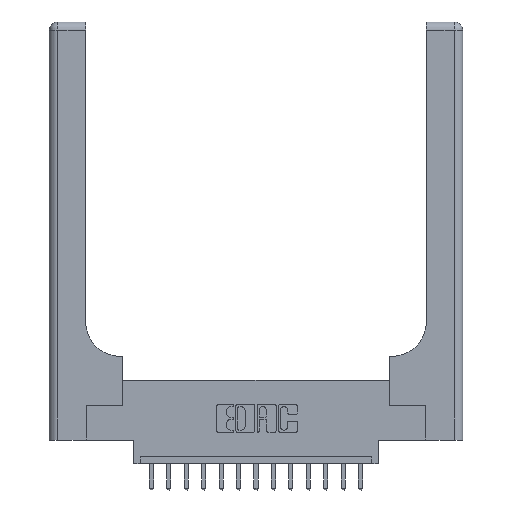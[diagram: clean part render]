
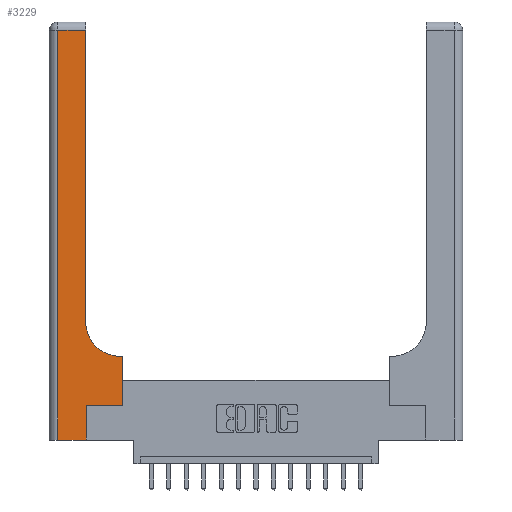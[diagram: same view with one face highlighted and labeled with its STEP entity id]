
A CAD part, top view. The second image highlights one B-rep face of the part: STEP entity #3229.
In plain terms, the highlighted planar face has unit normal (0, 0, 1).
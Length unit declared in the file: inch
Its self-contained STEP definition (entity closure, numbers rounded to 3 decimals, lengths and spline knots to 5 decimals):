
#94 = EDGE_CURVE ( 'NONE', #2724, #3836, #13927, .T. ) ;
#592 = ORIENTED_EDGE ( 'NONE', *, *, #8677, .T. ) ;
#662 = EDGE_CURVE ( 'NONE', #2136, #1271, #756, .T. ) ;
#756 = LINE ( 'NONE', #15656, #7373 ) ;
#809 = CARTESIAN_POINT ( 'NONE',  ( 0.265, 0.25, 0.37 ) ) ;
#1271 = VERTEX_POINT ( 'NONE', #15515 ) ;
#1373 = DIRECTION ( 'NONE',  ( 0., 1., 0. ) ) ;
#1915 = VERTEX_POINT ( 'NONE', #5885 ) ;
#1947 = VECTOR ( 'NONE', #14569, 39.37008 ) ;
#2000 = ORIENTED_EDGE ( 'NONE', *, *, #14840, .T. ) ;
#2136 = VERTEX_POINT ( 'NONE', #6318 ) ;
#2673 = ORIENTED_EDGE ( 'NONE', *, *, #662, .T. ) ;
#2724 = VERTEX_POINT ( 'NONE', #8294 ) ;
#2776 = EDGE_LOOP ( 'NONE', ( #4238, #15175, #2673, #2000, #15397, #592, #6553, #10457, #15063 ) ) ;
#3229 = ADVANCED_FACE ( 'NONE', ( #16634 ), #5889, .F. ) ;
#3540 = CARTESIAN_POINT ( 'NONE',  ( 0.528, 0.25, 0.37 ) ) ;
#3836 = VERTEX_POINT ( 'NONE', #5038 ) ;
#3899 = EDGE_CURVE ( 'NONE', #4764, #2724, #15065, .T. ) ;
#4098 = LINE ( 'NONE', #9790, #9730 ) ;
#4238 = ORIENTED_EDGE ( 'NONE', *, *, #11075, .T. ) ;
#4522 = DIRECTION ( 'NONE',  ( 0., 0., -1. ) ) ;
#4531 = DIRECTION ( 'NONE',  ( -1., 0., 0. ) ) ;
#4764 = VERTEX_POINT ( 'NONE', #15615 ) ;
#5038 = CARTESIAN_POINT ( 'NONE',  ( 0.26, 0.85, 0.37 ) ) ;
#5266 = AXIS2_PLACEMENT_3D ( 'NONE', #11491, #4522, #13010 ) ;
#5885 = CARTESIAN_POINT ( 'NONE',  ( 0.528, 0.25, 0.37 ) ) ;
#5889 = PLANE ( 'NONE',  #13922 ) ;
#6251 = DIRECTION ( 'NONE',  ( 0., -1., 0. ) ) ;
#6318 = CARTESIAN_POINT ( 'NONE',  ( 0.06, 2.94, 0.37 ) ) ;
#6520 = LINE ( 'NONE', #3540, #1947 ) ;
#6522 = CARTESIAN_POINT ( 'NONE',  ( 0.26, 2.94, 0.37 ) ) ;
#6553 = ORIENTED_EDGE ( 'NONE', *, *, #9746, .T. ) ;
#7241 = VERTEX_POINT ( 'NONE', #6522 ) ;
#7373 = VECTOR ( 'NONE', #6251, 39.37008 ) ;
#7734 = CARTESIAN_POINT ( 'NONE',  ( 0., 0., 0.37 ) ) ;
#7825 = VECTOR ( 'NONE', #15867, 39.37008 ) ;
#8101 = EDGE_CURVE ( 'NONE', #7241, #2136, #4098, .T. ) ;
#8294 = CARTESIAN_POINT ( 'NONE',  ( 0.51, 0.6, 0.37 ) ) ;
#8483 = DIRECTION ( 'NONE',  ( -1., 0., 0. ) ) ;
#8615 = CARTESIAN_POINT ( 'NONE',  ( 0.265, 0., 0.37 ) ) ;
#8677 = EDGE_CURVE ( 'NONE', #10561, #1915, #14022, .T. ) ;
#8700 = LINE ( 'NONE', #7734, #7825 ) ;
#9619 = DIRECTION ( 'NONE',  ( -1., 0., 0. ) ) ;
#9730 = VECTOR ( 'NONE', #9619, 39.37008 ) ;
#9746 = EDGE_CURVE ( 'NONE', #1915, #4764, #6520, .T. ) ;
#9790 = CARTESIAN_POINT ( 'NONE',  ( 0., 2.94, 0.37 ) ) ;
#10019 = VERTEX_POINT ( 'NONE', #8615 ) ;
#10326 = CARTESIAN_POINT ( 'NONE',  ( 0.26, 3., 0.37 ) ) ;
#10457 = ORIENTED_EDGE ( 'NONE', *, *, #3899, .T. ) ;
#10561 = VERTEX_POINT ( 'NONE', #809 ) ;
#10565 = VECTOR ( 'NONE', #12584, 39.37008 ) ;
#11075 = EDGE_CURVE ( 'NONE', #3836, #7241, #13382, .T. ) ;
#11117 = LINE ( 'NONE', #12571, #16758 ) ;
#11491 = CARTESIAN_POINT ( 'NONE',  ( 0.51, 0.85, 0.37 ) ) ;
#11771 = VECTOR ( 'NONE', #8483, 39.37008 ) ;
#12571 = CARTESIAN_POINT ( 'NONE',  ( 0.265, 0., 0.37 ) ) ;
#12584 = DIRECTION ( 'NONE',  ( 1., 0., 0. ) ) ;
#12679 = DIRECTION ( 'NONE',  ( 0., 0., -1. ) ) ;
#13010 = DIRECTION ( 'NONE',  ( 1., 0., 0. ) ) ;
#13382 = LINE ( 'NONE', #10326, #16382 ) ;
#13922 = AXIS2_PLACEMENT_3D ( 'NONE', #13933, #12679, #4531 ) ;
#13927 = CIRCLE ( 'NONE', #5266, 0.25 ) ;
#13933 = CARTESIAN_POINT ( 'NONE',  ( 0., 3., 0.37 ) ) ;
#14022 = LINE ( 'NONE', #15469, #10565 ) ;
#14569 = DIRECTION ( 'NONE',  ( 0., 1., 0. ) ) ;
#14840 = EDGE_CURVE ( 'NONE', #1271, #10019, #8700, .T. ) ;
#15063 = ORIENTED_EDGE ( 'NONE', *, *, #94, .T. ) ;
#15065 = LINE ( 'NONE', #15243, #11771 ) ;
#15175 = ORIENTED_EDGE ( 'NONE', *, *, #8101, .T. ) ;
#15243 = CARTESIAN_POINT ( 'NONE',  ( 0.26, 0.6, 0.37 ) ) ;
#15397 = ORIENTED_EDGE ( 'NONE', *, *, #16261, .T. ) ;
#15469 = CARTESIAN_POINT ( 'NONE',  ( 0.265, 0.25, 0.37 ) ) ;
#15515 = CARTESIAN_POINT ( 'NONE',  ( 0.06, 0., 0.37 ) ) ;
#15615 = CARTESIAN_POINT ( 'NONE',  ( 0.528, 0.6, 0.37 ) ) ;
#15656 = CARTESIAN_POINT ( 'NONE',  ( 0.06, 3., 0.37 ) ) ;
#15867 = DIRECTION ( 'NONE',  ( 1., 0., 0. ) ) ;
#16261 = EDGE_CURVE ( 'NONE', #10019, #10561, #11117, .T. ) ;
#16382 = VECTOR ( 'NONE', #17015, 39.37008 ) ;
#16634 = FACE_OUTER_BOUND ( 'NONE', #2776, .T. ) ;
#16758 = VECTOR ( 'NONE', #1373, 39.37008 ) ;
#17015 = DIRECTION ( 'NONE',  ( 0., 1., 0. ) ) ;
